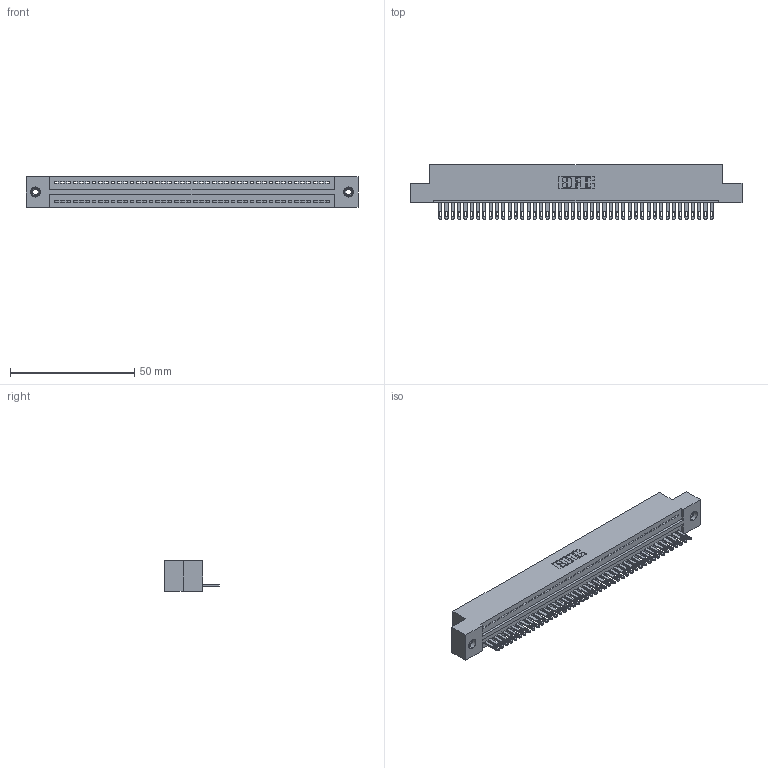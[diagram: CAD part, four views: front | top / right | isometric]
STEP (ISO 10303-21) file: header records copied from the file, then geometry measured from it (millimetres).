
FILE_DESCRIPTION (( 'STEP AP203' ), '1' );
FILE_NAME ('325-044-500-108.STEP', '2020-02-24T22:16:47', ( '' ), ( '' ), 'SwSTEP 2.0', 'SolidWorks 2016', '' );
FILE_SCHEMA (( 'CONFIG_CONTROL_DESIGN' ));
Length unit declared in the file: inch
Products named in the file (4): 345-250-001_345-250-003-102; 325-292-001_325-293-100; 325-044-500-108; 325 Part_TI
Assembly tree (47 placements, depth 2):
  325-044-500-108
    325 Part_TI
    325-292-001_325-293-100  x44
    345-250-001_345-250-003-102  x2
Bounding box: 133.48 x 21.84 x 12.45 mm (x, y, z)
Volume: 16981.5 mm3; surface area: 18704.6 mm2
Topology: 47 solids, 47 shells, 2550 faces, 7839 edges, 5218 vertices
Faces by surface type: plane 1686, cylinder 848, cone 12, torus 4
Entity records: 27756 total; most frequent: CARTESIAN_POINT 4769, ORIENTED_EDGE 4742, DIRECTION 4053, EDGE_CURVE 2371, LINE 2219, VECTOR 2219, VERTEX_POINT 1576, AXIS2_PLACEMENT_3D 917
